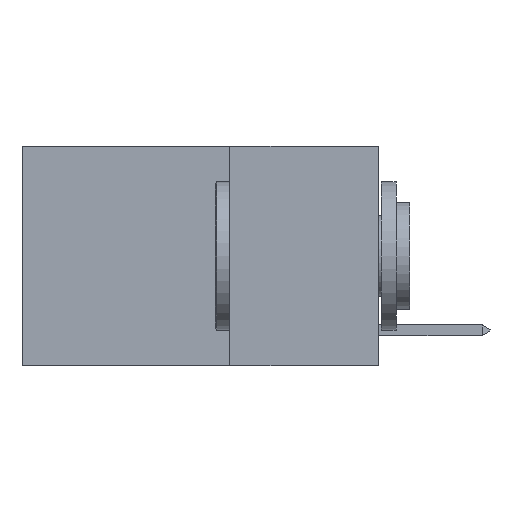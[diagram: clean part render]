
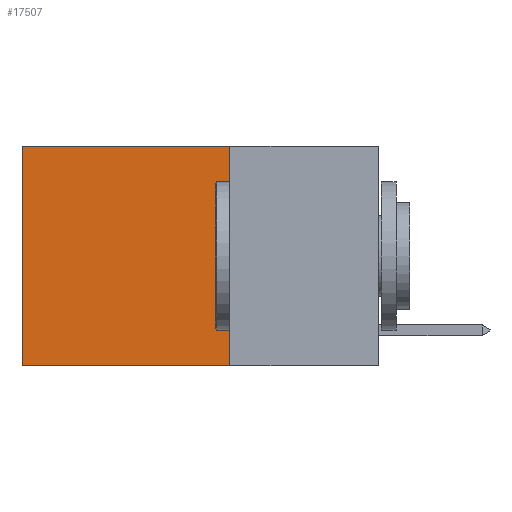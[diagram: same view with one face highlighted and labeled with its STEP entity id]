
A CAD part, left-side view. The second image highlights one B-rep face of the part: STEP entity #17507.
In plain terms, the highlighted planar face has unit normal (-1, 0, 0).
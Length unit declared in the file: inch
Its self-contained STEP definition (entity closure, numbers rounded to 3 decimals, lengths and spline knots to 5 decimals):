
#116 = DIRECTION ( 'NONE',  ( 0., 0., -1. ) ) ;
#1566 = CARTESIAN_POINT ( 'NONE',  ( 0.2625, 0.25, 0. ) ) ;
#2178 = VECTOR ( 'NONE', #19186, 39.37008 ) ;
#2221 = DIRECTION ( 'NONE',  ( 0., 0., -1. ) ) ;
#3159 = CARTESIAN_POINT ( 'NONE',  ( 0.2625, 0.25, 0. ) ) ;
#4434 = CARTESIAN_POINT ( 'NONE',  ( 0.2625, 0.25, -0.37 ) ) ;
#4521 = PLANE ( 'NONE',  #5148 ) ;
#5148 = AXIS2_PLACEMENT_3D ( 'NONE', #11363, #8115, #6257 ) ;
#5185 = VECTOR ( 'NONE', #22409, 39.37008 ) ;
#6257 = DIRECTION ( 'NONE',  ( 0., 0., -1. ) ) ;
#6820 = CARTESIAN_POINT ( 'NONE',  ( 0.2625, 0.25, -0.37 ) ) ;
#7553 = VERTEX_POINT ( 'NONE', #17363 ) ;
#8115 = DIRECTION ( 'NONE',  ( 1., 0., 0. ) ) ;
#8417 = LINE ( 'NONE', #1566, #5185 ) ;
#9345 = VERTEX_POINT ( 'NONE', #11349 ) ;
#9813 = VECTOR ( 'NONE', #116, 39.37008 ) ;
#10249 = VECTOR ( 'NONE', #2221, 39.37008 ) ;
#11349 = CARTESIAN_POINT ( 'NONE',  ( 0.2625, 0.6, 0. ) ) ;
#11363 = CARTESIAN_POINT ( 'NONE',  ( 0.2625, 0.25, 0. ) ) ;
#12345 = EDGE_LOOP ( 'NONE', ( #21789, #19104, #16368, #20039 ) ) ;
#12668 = LINE ( 'NONE', #17853, #10249 ) ;
#13737 = EDGE_CURVE ( 'NONE', #9345, #7553, #15986, .T. ) ;
#14096 = LINE ( 'NONE', #6820, #2178 ) ;
#15124 = EDGE_CURVE ( 'NONE', #17172, #17175, #12668, .T. ) ;
#15986 = LINE ( 'NONE', #19349, #9813 ) ;
#16368 = ORIENTED_EDGE ( 'NONE', *, *, #15124, .F. ) ;
#17138 = FACE_OUTER_BOUND ( 'NONE', #12345, .T. ) ;
#17172 = VERTEX_POINT ( 'NONE', #3159 ) ;
#17175 = VERTEX_POINT ( 'NONE', #4434 ) ;
#17363 = CARTESIAN_POINT ( 'NONE',  ( 0.2625, 0.6, -0.37 ) ) ;
#17507 = ADVANCED_FACE ( 'NONE', ( #17138 ), #4521, .F. ) ;
#17853 = CARTESIAN_POINT ( 'NONE',  ( 0.2625, 0.25, 0. ) ) ;
#19104 = ORIENTED_EDGE ( 'NONE', *, *, #19521, .F. ) ;
#19186 = DIRECTION ( 'NONE',  ( 0., 1., 0. ) ) ;
#19349 = CARTESIAN_POINT ( 'NONE',  ( 0.2625, 0.6, 0. ) ) ;
#19521 = EDGE_CURVE ( 'NONE', #17175, #7553, #14096, .T. ) ;
#19971 = EDGE_CURVE ( 'NONE', #17172, #9345, #8417, .T. ) ;
#20039 = ORIENTED_EDGE ( 'NONE', *, *, #19971, .T. ) ;
#21789 = ORIENTED_EDGE ( 'NONE', *, *, #13737, .T. ) ;
#22409 = DIRECTION ( 'NONE',  ( 0., 1., 0. ) ) ;
